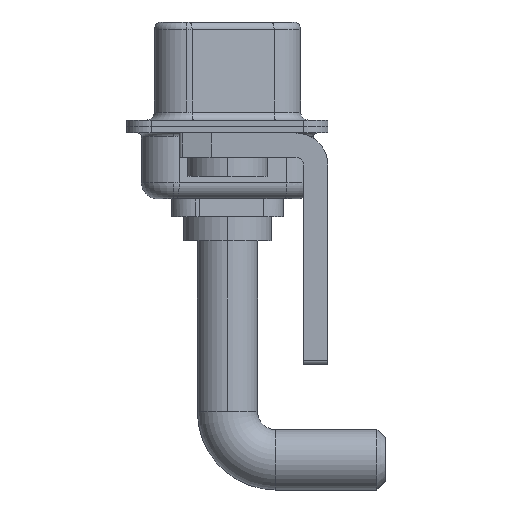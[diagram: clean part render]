
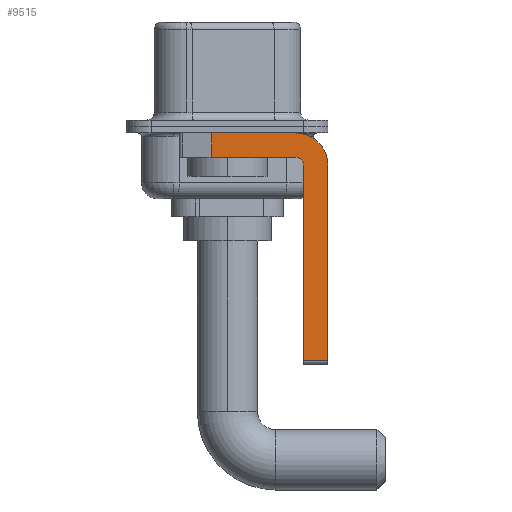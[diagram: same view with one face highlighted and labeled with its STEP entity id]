
A CAD part, left-side view. The second image highlights one B-rep face of the part: STEP entity #9515.
In plain terms, the highlighted planar face has unit normal (-1, 0, 0).
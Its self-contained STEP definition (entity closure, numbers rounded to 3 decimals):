
#1058 = VECTOR ( 'NONE', #6068, 1000. ) ;
#1433 = VERTEX_POINT ( 'NONE', #9529 ) ;
#1589 = FACE_OUTER_BOUND ( 'NONE', #2448, .T. ) ;
#1722 = EDGE_CURVE ( 'NONE', #13444, #14199, #16922, .T. ) ;
#1907 = DIRECTION ( 'NONE',  ( 0., 0., -1. ) ) ;
#1936 = AXIS2_PLACEMENT_3D ( 'NONE', #9278, #6856, #2878 ) ;
#2032 = LINE ( 'NONE', #8480, #10048 ) ;
#2335 = VECTOR ( 'NONE', #7111, 1000. ) ;
#2431 = DIRECTION ( 'NONE',  ( 0., -1., 0. ) ) ;
#2448 = EDGE_LOOP ( 'NONE', ( #14955, #12105, #13417, #13162, #15884, #13973, #13719, #7194 ) ) ;
#2793 = PLANE ( 'NONE',  #1936 ) ;
#2875 = LINE ( 'NONE', #11954, #14363 ) ;
#2878 = DIRECTION ( 'NONE',  ( 0., 0., -1. ) ) ;
#2929 = EDGE_CURVE ( 'NONE', #13159, #7373, #2875, .T. ) ;
#3302 = CARTESIAN_POINT ( 'NONE',  ( -2.9, -6.25, -14.55 ) ) ;
#3434 = CARTESIAN_POINT ( 'NONE',  ( -2.9, -4.25, -2.4 ) ) ;
#3860 = CARTESIAN_POINT ( 'NONE',  ( -2.9, -4.75, -14.55 ) ) ;
#4445 = CARTESIAN_POINT ( 'NONE',  ( -2.9, 0.978, -1.9 ) ) ;
#4472 = CARTESIAN_POINT ( 'NONE',  ( -2.9, -4.75, -2.4 ) ) ;
#5031 = EDGE_CURVE ( 'NONE', #7373, #6834, #9134, .T. ) ;
#5035 = CARTESIAN_POINT ( 'NONE',  ( -2.9, -6.25, -2.4 ) ) ;
#5159 = EDGE_CURVE ( 'NONE', #13159, #16078, #7637, .T. ) ;
#5356 = VECTOR ( 'NONE', #14133, 1000. ) ;
#5490 = DIRECTION ( 'NONE',  ( 0., 0., 1. ) ) ;
#5996 = DIRECTION ( 'NONE',  ( 0., 1., 0. ) ) ;
#6068 = DIRECTION ( 'NONE',  ( 0., 0., -1. ) ) ;
#6318 = CARTESIAN_POINT ( 'NONE',  ( -2.9, 3., -0.4 ) ) ;
#6834 = VERTEX_POINT ( 'NONE', #12266 ) ;
#6856 = DIRECTION ( 'NONE',  ( 1., 0., 0. ) ) ;
#6900 = EDGE_CURVE ( 'NONE', #14199, #1433, #14296, .T. ) ;
#7111 = DIRECTION ( 'NONE',  ( 0., 0., -1. ) ) ;
#7194 = ORIENTED_EDGE ( 'NONE', *, *, #6900, .F. ) ;
#7373 = VERTEX_POINT ( 'NONE', #4472 ) ;
#7520 = CARTESIAN_POINT ( 'NONE',  ( -2.9, 0.978, -1.9 ) ) ;
#7637 = LINE ( 'NONE', #14040, #5356 ) ;
#8470 = EDGE_CURVE ( 'NONE', #1433, #16078, #16834, .T. ) ;
#8480 = CARTESIAN_POINT ( 'NONE',  ( -2.9, -4.25, -1.9 ) ) ;
#9134 = CIRCLE ( 'NONE', #15448, 0.5 ) ;
#9278 = CARTESIAN_POINT ( 'NONE',  ( -2.9, -4.25, -2.4 ) ) ;
#9515 = ADVANCED_FACE ( 'NONE', ( #1589 ), #2793, .F. ) ;
#9529 = CARTESIAN_POINT ( 'NONE',  ( -2.9, -6.25, -2.4 ) ) ;
#10048 = VECTOR ( 'NONE', #5996, 1000. ) ;
#11445 = DIRECTION ( 'NONE',  ( 0., 0., 1. ) ) ;
#11535 = CARTESIAN_POINT ( 'NONE',  ( -2.9, -4.25, -0.4 ) ) ;
#11842 = VECTOR ( 'NONE', #2431, 1000. ) ;
#11954 = CARTESIAN_POINT ( 'NONE',  ( -2.9, -4.75, -14.8 ) ) ;
#12105 = ORIENTED_EDGE ( 'NONE', *, *, #16109, .T. ) ;
#12266 = CARTESIAN_POINT ( 'NONE',  ( -2.9, -4.25, -1.9 ) ) ;
#13012 = VERTEX_POINT ( 'NONE', #7520 ) ;
#13159 = VERTEX_POINT ( 'NONE', #3860 ) ;
#13162 = ORIENTED_EDGE ( 'NONE', *, *, #5031, .F. ) ;
#13417 = ORIENTED_EDGE ( 'NONE', *, *, #16115, .F. ) ;
#13444 = VERTEX_POINT ( 'NONE', #14445 ) ;
#13719 = ORIENTED_EDGE ( 'NONE', *, *, #8470, .F. ) ;
#13956 = CARTESIAN_POINT ( 'NONE',  ( -2.9, -4.25, -2.4 ) ) ;
#13973 = ORIENTED_EDGE ( 'NONE', *, *, #5159, .T. ) ;
#14040 = CARTESIAN_POINT ( 'NONE',  ( -2.9, -4.25, -14.55 ) ) ;
#14133 = DIRECTION ( 'NONE',  ( 0., -1., 0. ) ) ;
#14199 = VERTEX_POINT ( 'NONE', #11535 ) ;
#14296 = CIRCLE ( 'NONE', #16756, 2. ) ;
#14363 = VECTOR ( 'NONE', #5490, 1000. ) ;
#14445 = CARTESIAN_POINT ( 'NONE',  ( -2.9, 0.978, -0.4 ) ) ;
#14955 = ORIENTED_EDGE ( 'NONE', *, *, #1722, .F. ) ;
#15133 = LINE ( 'NONE', #4445, #2335 ) ;
#15182 = DIRECTION ( 'NONE',  ( 1., 0., 0. ) ) ;
#15247 = DIRECTION ( 'NONE',  ( -1., 0., 0. ) ) ;
#15448 = AXIS2_PLACEMENT_3D ( 'NONE', #13956, #15247, #11445 ) ;
#15884 = ORIENTED_EDGE ( 'NONE', *, *, #2929, .F. ) ;
#16078 = VERTEX_POINT ( 'NONE', #3302 ) ;
#16109 = EDGE_CURVE ( 'NONE', #13444, #13012, #15133, .T. ) ;
#16115 = EDGE_CURVE ( 'NONE', #6834, #13012, #2032, .T. ) ;
#16756 = AXIS2_PLACEMENT_3D ( 'NONE', #3434, #15182, #1907 ) ;
#16834 = LINE ( 'NONE', #5035, #1058 ) ;
#16922 = LINE ( 'NONE', #6318, #11842 ) ;
